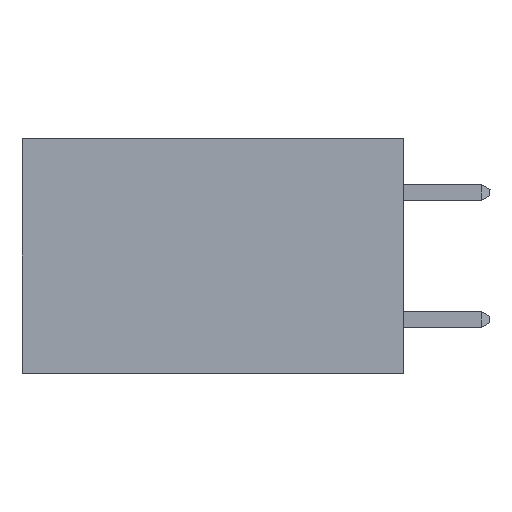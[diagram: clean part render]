
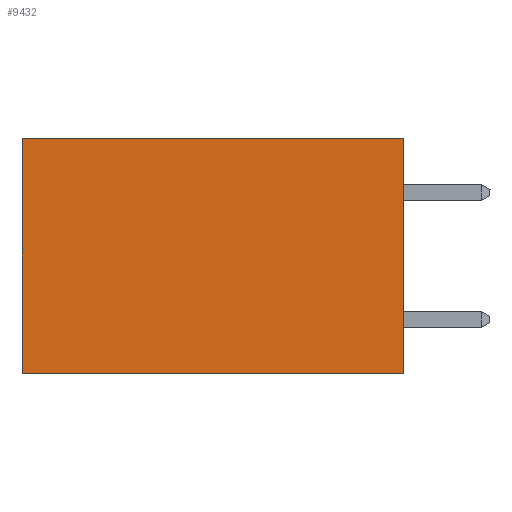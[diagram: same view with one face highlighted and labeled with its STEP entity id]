
A CAD part, left-side view. The second image highlights one B-rep face of the part: STEP entity #9432.
In plain terms, the highlighted planar face has unit normal (-1, 0, 0).
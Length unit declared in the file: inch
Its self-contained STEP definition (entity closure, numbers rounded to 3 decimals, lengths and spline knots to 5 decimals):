
#260 = PLANE ( 'NONE',  #6967 ) ;
#393 = CARTESIAN_POINT ( 'NONE',  ( 0.2875, 0., 0. ) ) ;
#1186 = ORIENTED_EDGE ( 'NONE', *, *, #13408, .F. ) ;
#2711 = LINE ( 'NONE', #393, #23292 ) ;
#3971 = DIRECTION ( 'NONE',  ( 0., 0., -1. ) ) ;
#5032 = CARTESIAN_POINT ( 'NONE',  ( 0.2875, 0., 0. ) ) ;
#5396 = EDGE_LOOP ( 'NONE', ( #16961, #12881, #1186, #10786 ) ) ;
#6768 = EDGE_CURVE ( 'NONE', #17408, #17682, #20791, .T. ) ;
#6834 = EDGE_CURVE ( 'NONE', #15482, #17408, #23970, .T. ) ;
#6967 = AXIS2_PLACEMENT_3D ( 'NONE', #22727, #15226, #3971 ) ;
#8908 = FACE_OUTER_BOUND ( 'NONE', #5396, .T. ) ;
#9432 = ADVANCED_FACE ( 'NONE', ( #8908 ), #260, .F. ) ;
#10539 = CARTESIAN_POINT ( 'NONE',  ( 0.2875, 0.6, 0. ) ) ;
#10786 = ORIENTED_EDGE ( 'NONE', *, *, #6834, .T. ) ;
#12644 = DIRECTION ( 'NONE',  ( 0., 1., 0. ) ) ;
#12881 = ORIENTED_EDGE ( 'NONE', *, *, #21952, .F. ) ;
#13408 = EDGE_CURVE ( 'NONE', #15482, #24169, #2711, .T. ) ;
#13435 = DIRECTION ( 'NONE',  ( 0., 0., -1. ) ) ;
#13956 = VECTOR ( 'NONE', #14473, 39.37008 ) ;
#14473 = DIRECTION ( 'NONE',  ( 0., 1., 0. ) ) ;
#14653 = LINE ( 'NONE', #18386, #20282 ) ;
#15058 = CARTESIAN_POINT ( 'NONE',  ( 0.2875, 0.6, -0.37 ) ) ;
#15226 = DIRECTION ( 'NONE',  ( 1., 0., 0. ) ) ;
#15482 = VERTEX_POINT ( 'NONE', #15504 ) ;
#15504 = CARTESIAN_POINT ( 'NONE',  ( 0.2875, 0., 0. ) ) ;
#15617 = CARTESIAN_POINT ( 'NONE',  ( 0.2875, 0., -0.37 ) ) ;
#16961 = ORIENTED_EDGE ( 'NONE', *, *, #6768, .T. ) ;
#17408 = VERTEX_POINT ( 'NONE', #18012 ) ;
#17682 = VERTEX_POINT ( 'NONE', #15058 ) ;
#18012 = CARTESIAN_POINT ( 'NONE',  ( 0.2875, 0.6, 0. ) ) ;
#18386 = CARTESIAN_POINT ( 'NONE',  ( 0.2875, 0., -0.37 ) ) ;
#20282 = VECTOR ( 'NONE', #12644, 39.37008 ) ;
#20791 = LINE ( 'NONE', #10539, #21362 ) ;
#21362 = VECTOR ( 'NONE', #23617, 39.37008 ) ;
#21952 = EDGE_CURVE ( 'NONE', #24169, #17682, #14653, .T. ) ;
#22727 = CARTESIAN_POINT ( 'NONE',  ( 0.2875, 0., 0. ) ) ;
#23292 = VECTOR ( 'NONE', #13435, 39.37008 ) ;
#23617 = DIRECTION ( 'NONE',  ( 0., 0., -1. ) ) ;
#23970 = LINE ( 'NONE', #5032, #13956 ) ;
#24169 = VERTEX_POINT ( 'NONE', #15617 ) ;
